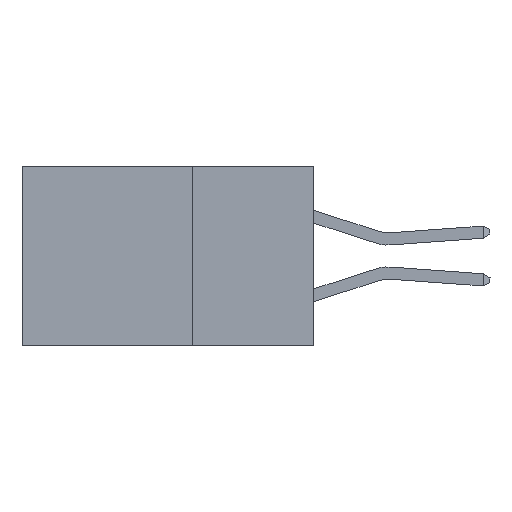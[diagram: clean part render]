
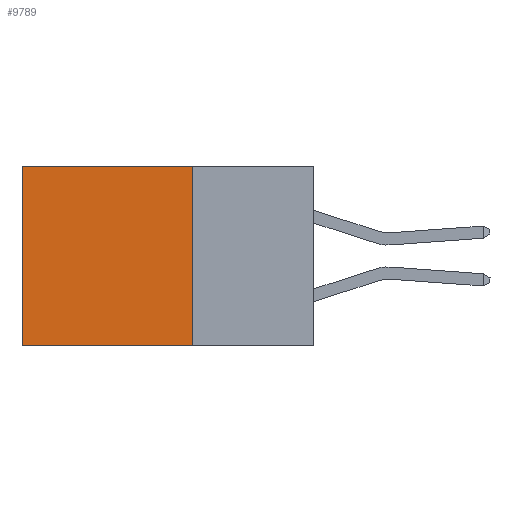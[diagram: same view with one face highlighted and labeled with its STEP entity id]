
A CAD part, left-side view. The second image highlights one B-rep face of the part: STEP entity #9789.
In plain terms, the highlighted planar face has unit normal (-1, 0, 0).
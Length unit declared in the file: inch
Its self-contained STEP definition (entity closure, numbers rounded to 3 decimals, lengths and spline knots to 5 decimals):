
#1376 = VECTOR ( 'NONE', #11675, 39.37008 ) ;
#2653 = LINE ( 'NONE', #3637, #4693 ) ;
#2915 = EDGE_LOOP ( 'NONE', ( #22502, #11941, #23728, #13998 ) ) ;
#3007 = CARTESIAN_POINT ( 'NONE',  ( 0.2875, 0.6, -0.37 ) ) ;
#3637 = CARTESIAN_POINT ( 'NONE',  ( 0.2875, 0.25, 0. ) ) ;
#3974 = LINE ( 'NONE', #10290, #18400 ) ;
#4693 = VECTOR ( 'NONE', #5638, 39.37008 ) ;
#5317 = DIRECTION ( 'NONE',  ( 0., 1., 0. ) ) ;
#5468 = DIRECTION ( 'NONE',  ( 1., 0., 0. ) ) ;
#5638 = DIRECTION ( 'NONE',  ( 0., 1., 0. ) ) ;
#7601 = PLANE ( 'NONE',  #16444 ) ;
#7662 = VERTEX_POINT ( 'NONE', #23387 ) ;
#8055 = EDGE_CURVE ( 'NONE', #25935, #7662, #2653, .T. ) ;
#8928 = EDGE_CURVE ( 'NONE', #25935, #10390, #3974, .T. ) ;
#9701 = VECTOR ( 'NONE', #5317, 39.37008 ) ;
#9789 = ADVANCED_FACE ( 'NONE', ( #11303 ), #7601, .F. ) ;
#9856 = CARTESIAN_POINT ( 'NONE',  ( 0.2875, 0.25, 0. ) ) ;
#10290 = CARTESIAN_POINT ( 'NONE',  ( 0.2875, 0.25, 0. ) ) ;
#10390 = VERTEX_POINT ( 'NONE', #19954 ) ;
#10900 = EDGE_CURVE ( 'NONE', #10390, #15949, #21800, .T. ) ;
#11303 = FACE_OUTER_BOUND ( 'NONE', #2915, .T. ) ;
#11675 = DIRECTION ( 'NONE',  ( 0., 0., -1. ) ) ;
#11717 = DIRECTION ( 'NONE',  ( 0., 0., -1. ) ) ;
#11941 = ORIENTED_EDGE ( 'NONE', *, *, #10900, .F. ) ;
#13998 = ORIENTED_EDGE ( 'NONE', *, *, #8055, .T. ) ;
#15814 = CARTESIAN_POINT ( 'NONE',  ( 0.2875, 0.6, 0. ) ) ;
#15949 = VERTEX_POINT ( 'NONE', #3007 ) ;
#16444 = AXIS2_PLACEMENT_3D ( 'NONE', #9856, #5468, #11717 ) ;
#17123 = DIRECTION ( 'NONE',  ( 0., 0., -1. ) ) ;
#18400 = VECTOR ( 'NONE', #17123, 39.37008 ) ;
#19954 = CARTESIAN_POINT ( 'NONE',  ( 0.2875, 0.25, -0.37 ) ) ;
#21219 = LINE ( 'NONE', #15814, #1376 ) ;
#21800 = LINE ( 'NONE', #26483, #9701 ) ;
#22502 = ORIENTED_EDGE ( 'NONE', *, *, #24251, .T. ) ;
#23387 = CARTESIAN_POINT ( 'NONE',  ( 0.2875, 0.6, 0. ) ) ;
#23728 = ORIENTED_EDGE ( 'NONE', *, *, #8928, .F. ) ;
#24251 = EDGE_CURVE ( 'NONE', #7662, #15949, #21219, .T. ) ;
#25935 = VERTEX_POINT ( 'NONE', #26453 ) ;
#26453 = CARTESIAN_POINT ( 'NONE',  ( 0.2875, 0.25, 0. ) ) ;
#26483 = CARTESIAN_POINT ( 'NONE',  ( 0.2875, 0.25, -0.37 ) ) ;
